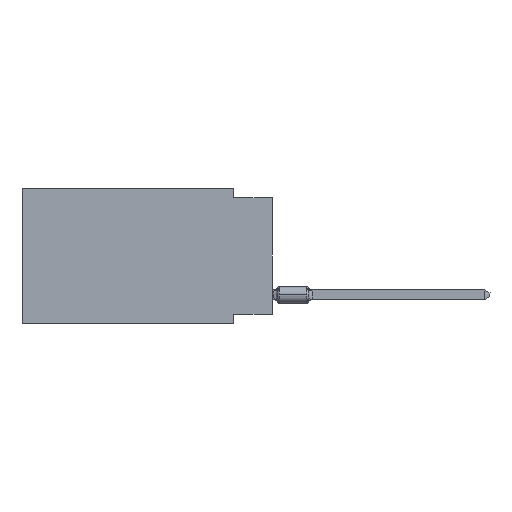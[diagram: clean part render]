
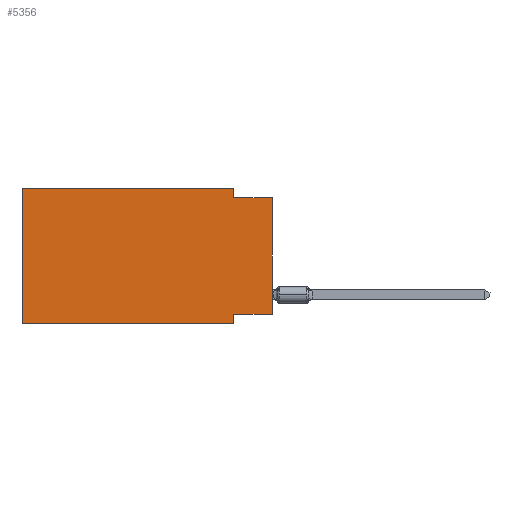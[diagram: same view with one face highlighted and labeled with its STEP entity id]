
A CAD part, left-side view. The second image highlights one B-rep face of the part: STEP entity #5356.
In plain terms, the highlighted planar face has unit normal (-1, 0, 0).
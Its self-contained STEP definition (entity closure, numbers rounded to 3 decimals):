
#443 = VERTEX_POINT ( 'NONE', #22703 ) ;
#785 = LINE ( 'NONE', #15494, #25309 ) ;
#1267 = CARTESIAN_POINT ( 'NONE',  ( 0., 16.383, 0. ) ) ;
#1575 = EDGE_CURVE ( 'NONE', #14684, #3260, #6315, .T. ) ;
#1639 = LINE ( 'NONE', #18278, #11646 ) ;
#2047 = CARTESIAN_POINT ( 'NONE',  ( 0., 16.383, 0. ) ) ;
#2207 = ORIENTED_EDGE ( 'NONE', *, *, #5720, .F. ) ;
#2479 = DIRECTION ( 'NONE',  ( 0., 0., 1. ) ) ;
#2735 = PLANE ( 'NONE',  #20048 ) ;
#2860 = CARTESIAN_POINT ( 'NONE',  ( 0., 16.383, 0. ) ) ;
#3084 = VERTEX_POINT ( 'NONE', #21457 ) ;
#3134 = DIRECTION ( 'NONE',  ( 0., 0., -1. ) ) ;
#3260 = VERTEX_POINT ( 'NONE', #1267 ) ;
#4476 = ORIENTED_EDGE ( 'NONE', *, *, #11814, .F. ) ;
#5131 = DIRECTION ( 'NONE',  ( 0., -1., 0. ) ) ;
#5285 = EDGE_CURVE ( 'NONE', #3084, #26059, #14722, .T. ) ;
#5356 = ADVANCED_FACE ( 'NONE', ( #19902 ), #2735, .F. ) ;
#5720 = EDGE_CURVE ( 'NONE', #26059, #26464, #785, .T. ) ;
#6174 = VERTEX_POINT ( 'NONE', #20414 ) ;
#6295 = VECTOR ( 'NONE', #18893, 1000. ) ;
#6315 = LINE ( 'NONE', #19520, #15250 ) ;
#6592 = VERTEX_POINT ( 'NONE', #9055 ) ;
#6790 = CARTESIAN_POINT ( 'NONE',  ( 0., 2.54, -8.89 ) ) ;
#6950 = LINE ( 'NONE', #23058, #10110 ) ;
#7611 = EDGE_LOOP ( 'NONE', ( #7928, #2207, #23605, #19253, #9162, #25639, #4476, #16227 ) ) ;
#7928 = ORIENTED_EDGE ( 'NONE', *, *, #26375, .T. ) ;
#8170 = LINE ( 'NONE', #6790, #20482 ) ;
#9055 = CARTESIAN_POINT ( 'NONE',  ( 0., 0., -8.255 ) ) ;
#9162 = ORIENTED_EDGE ( 'NONE', *, *, #1575, .F. ) ;
#9926 = CARTESIAN_POINT ( 'NONE',  ( 0., 0., 0. ) ) ;
#10110 = VECTOR ( 'NONE', #21544, 1000. ) ;
#10236 = DIRECTION ( 'NONE',  ( 0., -1., 0. ) ) ;
#11027 = DIRECTION ( 'NONE',  ( 1., 0., 0. ) ) ;
#11169 = VECTOR ( 'NONE', #10236, 1000. ) ;
#11646 = VECTOR ( 'NONE', #20469, 1000. ) ;
#11814 = EDGE_CURVE ( 'NONE', #6174, #443, #8170, .T. ) ;
#11994 = LINE ( 'NONE', #2047, #11169 ) ;
#14684 = VERTEX_POINT ( 'NONE', #18229 ) ;
#14722 = LINE ( 'NONE', #23056, #23519 ) ;
#15250 = VECTOR ( 'NONE', #2479, 1000. ) ;
#15494 = CARTESIAN_POINT ( 'NONE',  ( 0., 0., -0.635 ) ) ;
#15922 = CARTESIAN_POINT ( 'NONE',  ( 0., 0., -0.635 ) ) ;
#16227 = ORIENTED_EDGE ( 'NONE', *, *, #23880, .F. ) ;
#17048 = DIRECTION ( 'NONE',  ( 0., 0., -1. ) ) ;
#17974 = EDGE_CURVE ( 'NONE', #14684, #443, #1639, .T. ) ;
#18229 = CARTESIAN_POINT ( 'NONE',  ( 0., 16.383, -8.89 ) ) ;
#18278 = CARTESIAN_POINT ( 'NONE',  ( 0., 16.383, -8.89 ) ) ;
#18519 = EDGE_CURVE ( 'NONE', #3260, #3084, #11994, .T. ) ;
#18893 = DIRECTION ( 'NONE',  ( 0., 0., 1. ) ) ;
#19253 = ORIENTED_EDGE ( 'NONE', *, *, #18519, .F. ) ;
#19520 = CARTESIAN_POINT ( 'NONE',  ( 0., 16.383, 0. ) ) ;
#19902 = FACE_OUTER_BOUND ( 'NONE', #7611, .T. ) ;
#20039 = LINE ( 'NONE', #9926, #6295 ) ;
#20048 = AXIS2_PLACEMENT_3D ( 'NONE', #2860, #11027, #3134 ) ;
#20414 = CARTESIAN_POINT ( 'NONE',  ( 0., 2.54, -8.255 ) ) ;
#20469 = DIRECTION ( 'NONE',  ( 0., -1., 0. ) ) ;
#20482 = VECTOR ( 'NONE', #21129, 1000. ) ;
#21129 = DIRECTION ( 'NONE',  ( 0., 0., -1. ) ) ;
#21457 = CARTESIAN_POINT ( 'NONE',  ( 0., 2.54, 0. ) ) ;
#21544 = DIRECTION ( 'NONE',  ( 0., 1., 0. ) ) ;
#22703 = CARTESIAN_POINT ( 'NONE',  ( 0., 2.54, -8.89 ) ) ;
#23056 = CARTESIAN_POINT ( 'NONE',  ( 0., 2.54, 0. ) ) ;
#23058 = CARTESIAN_POINT ( 'NONE',  ( 0., 0., -8.255 ) ) ;
#23519 = VECTOR ( 'NONE', #17048, 1000. ) ;
#23605 = ORIENTED_EDGE ( 'NONE', *, *, #5285, .F. ) ;
#23880 = EDGE_CURVE ( 'NONE', #6592, #6174, #6950, .T. ) ;
#25309 = VECTOR ( 'NONE', #5131, 1000. ) ;
#25350 = CARTESIAN_POINT ( 'NONE',  ( 0., 2.54, -0.635 ) ) ;
#25639 = ORIENTED_EDGE ( 'NONE', *, *, #17974, .T. ) ;
#26059 = VERTEX_POINT ( 'NONE', #25350 ) ;
#26375 = EDGE_CURVE ( 'NONE', #6592, #26464, #20039, .T. ) ;
#26464 = VERTEX_POINT ( 'NONE', #15922 ) ;
